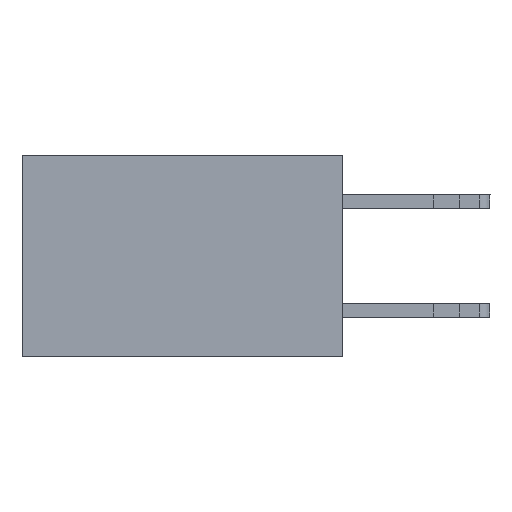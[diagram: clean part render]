
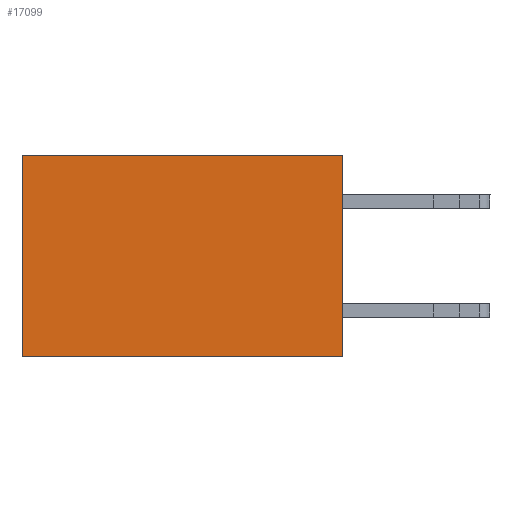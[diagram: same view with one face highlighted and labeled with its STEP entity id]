
A CAD part, left-side view. The second image highlights one B-rep face of the part: STEP entity #17099.
In plain terms, the highlighted planar face has unit normal (-1, 0, 0).
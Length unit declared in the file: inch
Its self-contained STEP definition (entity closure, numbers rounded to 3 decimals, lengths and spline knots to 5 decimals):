
#115 = CARTESIAN_POINT ( 'NONE',  ( 0.277, 0.59, -0.37 ) ) ;
#571 = EDGE_LOOP ( 'NONE', ( #12540, #11494, #9712, #7001 ) ) ;
#1545 = LINE ( 'NONE', #1656, #17957 ) ;
#1656 = CARTESIAN_POINT ( 'NONE',  ( 0.277, 0.59, -0.37 ) ) ;
#2740 = EDGE_CURVE ( 'NONE', #6216, #13064, #10298, .T. ) ;
#2909 = DIRECTION ( 'NONE',  ( 1., 0., 0. ) ) ;
#3529 = CARTESIAN_POINT ( 'NONE',  ( 0.277, 0., -0.37 ) ) ;
#4870 = VECTOR ( 'NONE', #19189, 39.37008 ) ;
#4920 = EDGE_CURVE ( 'NONE', #15185, #13485, #1545, .T. ) ;
#6216 = VERTEX_POINT ( 'NONE', #8904 ) ;
#6487 = PLANE ( 'NONE',  #8700 ) ;
#7001 = ORIENTED_EDGE ( 'NONE', *, *, #8379, .T. ) ;
#8100 = CARTESIAN_POINT ( 'NONE',  ( 0.277, 0., 0. ) ) ;
#8212 = LINE ( 'NONE', #8100, #20339 ) ;
#8379 = EDGE_CURVE ( 'NONE', #6216, #15185, #8212, .T. ) ;
#8700 = AXIS2_PLACEMENT_3D ( 'NONE', #13714, #2909, #10149 ) ;
#8904 = CARTESIAN_POINT ( 'NONE',  ( 0.277, 0., 0. ) ) ;
#9712 = ORIENTED_EDGE ( 'NONE', *, *, #2740, .F. ) ;
#10149 = DIRECTION ( 'NONE',  ( 0., 0., -1. ) ) ;
#10298 = LINE ( 'NONE', #12310, #14294 ) ;
#10464 = DIRECTION ( 'NONE',  ( 0., 0., -1. ) ) ;
#11494 = ORIENTED_EDGE ( 'NONE', *, *, #14655, .F. ) ;
#11929 = CARTESIAN_POINT ( 'NONE',  ( 0.277, 0.59, 0. ) ) ;
#12310 = CARTESIAN_POINT ( 'NONE',  ( 0.277, 0., -0.37 ) ) ;
#12540 = ORIENTED_EDGE ( 'NONE', *, *, #4920, .T. ) ;
#13064 = VERTEX_POINT ( 'NONE', #3529 ) ;
#13485 = VERTEX_POINT ( 'NONE', #115 ) ;
#13497 = CARTESIAN_POINT ( 'NONE',  ( 0.277, 0., -0.37 ) ) ;
#13714 = CARTESIAN_POINT ( 'NONE',  ( 0.277, 0., -0.37 ) ) ;
#14294 = VECTOR ( 'NONE', #14330, 39.37008 ) ;
#14330 = DIRECTION ( 'NONE',  ( 0., 0., -1. ) ) ;
#14655 = EDGE_CURVE ( 'NONE', #13064, #13485, #15612, .T. ) ;
#15185 = VERTEX_POINT ( 'NONE', #11929 ) ;
#15612 = LINE ( 'NONE', #13497, #4870 ) ;
#17099 = ADVANCED_FACE ( 'NONE', ( #22764 ), #6487, .F. ) ;
#17957 = VECTOR ( 'NONE', #10464, 39.37008 ) ;
#19189 = DIRECTION ( 'NONE',  ( 0., 1., 0. ) ) ;
#20339 = VECTOR ( 'NONE', #20931, 39.37008 ) ;
#20931 = DIRECTION ( 'NONE',  ( 0., 1., 0. ) ) ;
#22764 = FACE_OUTER_BOUND ( 'NONE', #571, .T. ) ;
